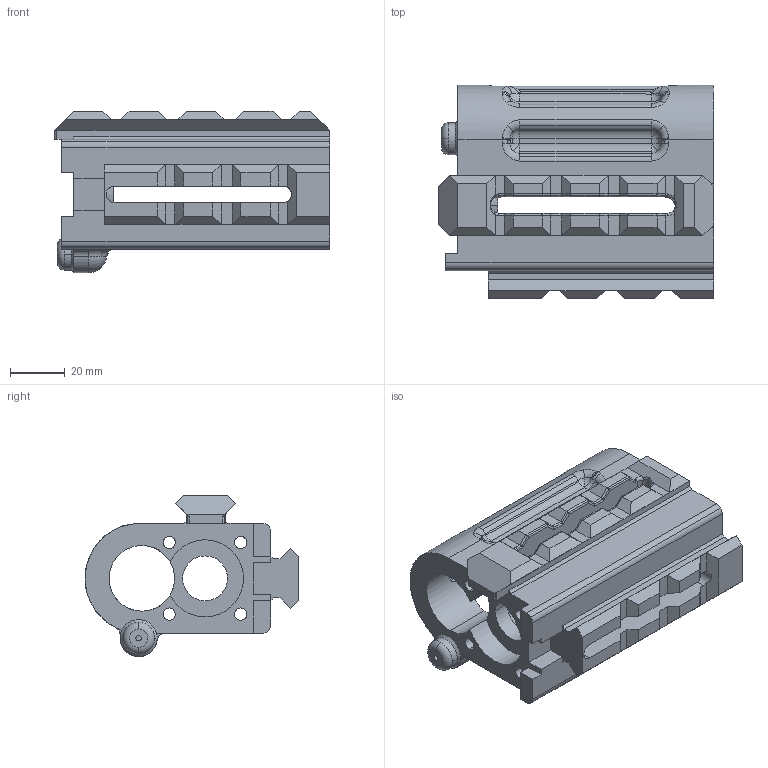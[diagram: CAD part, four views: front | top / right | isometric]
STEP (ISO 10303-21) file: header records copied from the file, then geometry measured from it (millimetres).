
FILE_DESCRIPTION(('STEP AP214'),'1');
FILE_NAME('WTF-9MVE BARREL RETAINER.stp','2020-09-01T22:11:50',(' '),(' '),'Spatial InterOp 3D',' ',' ');
FILE_SCHEMA(('AUTOMOTIVE_DESIGN { 1 0 10303 214 1 1 1 1 }'));
Length unit declared in the file: metre
Products named in the file (1): Solid
Bounding box: 100.82 x 78.16 x 59.03 mm (x, y, z)
Volume: 147371.6 mm3; surface area: 51460.1 mm2
Topology: 1 solids, 1 shells, 466 faces, 1218 edges, 751 vertices
Faces by surface type: cylinder 196, plane 131, torus 98, sphere 28, bspline 7, cone 6
Entity records: 17949 total; most frequent: CARTESIAN_POINT 6487, ORIENTED_EDGE 2432, DIRECTION 2422, EDGE_CURVE 1216, AXIS2_PLACEMENT_3D 941, VERTEX_POINT 747, LINE 540, VECTOR 540
